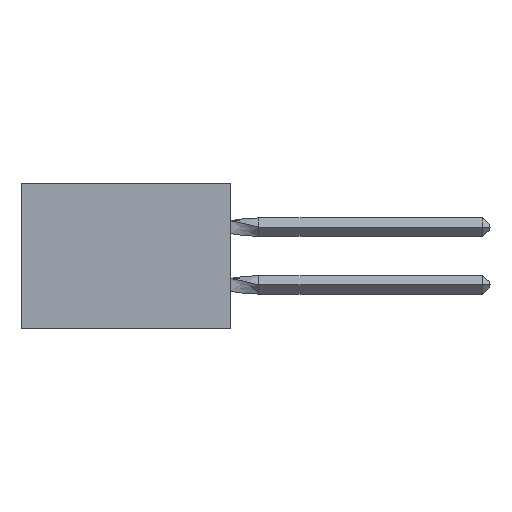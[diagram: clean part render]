
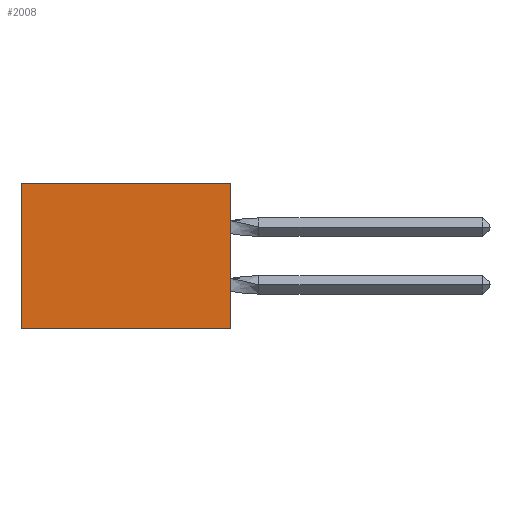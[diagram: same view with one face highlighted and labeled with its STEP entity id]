
A CAD part, left-side view. The second image highlights one B-rep face of the part: STEP entity #2008.
In plain terms, the highlighted planar face has unit normal (-1, 0, 0).
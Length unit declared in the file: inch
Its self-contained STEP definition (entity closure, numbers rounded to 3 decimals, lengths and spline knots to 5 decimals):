
#2 = EDGE_CURVE ( 'NONE', #4882, #5133, #2308, .T. ) ;
#170 = EDGE_CURVE ( 'NONE', #15903, #2973, #19072, .T. ) ;
#1425 = PLANE ( 'NONE',  #6571 ) ;
#1609 = DIRECTION ( 'NONE',  ( 0., 1., 0. ) ) ;
#1734 = EDGE_LOOP ( 'NONE', ( #16244, #10320, #10234, #14737 ) ) ;
#2008 = ADVANCED_FACE ( 'NONE', ( #11376 ), #1425, .F. ) ;
#2099 = CARTESIAN_POINT ( 'NONE',  ( 0.305, 0., 0. ) ) ;
#2308 = LINE ( 'NONE', #7234, #12898 ) ;
#2691 = DIRECTION ( 'NONE',  ( 1., 0., 0. ) ) ;
#2973 = VERTEX_POINT ( 'NONE', #13032 ) ;
#4241 = DIRECTION ( 'NONE',  ( 0., 0., -1. ) ) ;
#4315 = VECTOR ( 'NONE', #1609, 39.37008 ) ;
#4400 = DIRECTION ( 'NONE',  ( 0., 0., -1. ) ) ;
#4636 = CARTESIAN_POINT ( 'NONE',  ( 0.305, 0., -0.5 ) ) ;
#4882 = VERTEX_POINT ( 'NONE', #2099 ) ;
#5133 = VERTEX_POINT ( 'NONE', #4636 ) ;
#6571 = AXIS2_PLACEMENT_3D ( 'NONE', #17940, #2691, #4241 ) ;
#6821 = VECTOR ( 'NONE', #17662, 39.37008 ) ;
#7234 = CARTESIAN_POINT ( 'NONE',  ( 0.305, 0., -0.5 ) ) ;
#8200 = LINE ( 'NONE', #10620, #4315 ) ;
#10234 = ORIENTED_EDGE ( 'NONE', *, *, #2, .F. ) ;
#10320 = ORIENTED_EDGE ( 'NONE', *, *, #18420, .F. ) ;
#10620 = CARTESIAN_POINT ( 'NONE',  ( 0.305, 0., -0.5 ) ) ;
#11376 = FACE_OUTER_BOUND ( 'NONE', #1734, .T. ) ;
#12898 = VECTOR ( 'NONE', #16287, 39.37008 ) ;
#13032 = CARTESIAN_POINT ( 'NONE',  ( 0.305, 0.72, -0.5 ) ) ;
#13313 = EDGE_CURVE ( 'NONE', #4882, #15903, #15642, .T. ) ;
#14202 = CARTESIAN_POINT ( 'NONE',  ( 0.305, 0.72, 0. ) ) ;
#14737 = ORIENTED_EDGE ( 'NONE', *, *, #13313, .T. ) ;
#15642 = LINE ( 'NONE', #15879, #6821 ) ;
#15879 = CARTESIAN_POINT ( 'NONE',  ( 0.305, 0., 0. ) ) ;
#15903 = VERTEX_POINT ( 'NONE', #14202 ) ;
#16244 = ORIENTED_EDGE ( 'NONE', *, *, #170, .T. ) ;
#16287 = DIRECTION ( 'NONE',  ( 0., 0., -1. ) ) ;
#17662 = DIRECTION ( 'NONE',  ( 0., 1., 0. ) ) ;
#17940 = CARTESIAN_POINT ( 'NONE',  ( 0.305, 0., -0.5 ) ) ;
#18247 = CARTESIAN_POINT ( 'NONE',  ( 0.305, 0.72, -0.5 ) ) ;
#18420 = EDGE_CURVE ( 'NONE', #5133, #2973, #8200, .T. ) ;
#18850 = VECTOR ( 'NONE', #4400, 39.37008 ) ;
#19072 = LINE ( 'NONE', #18247, #18850 ) ;
